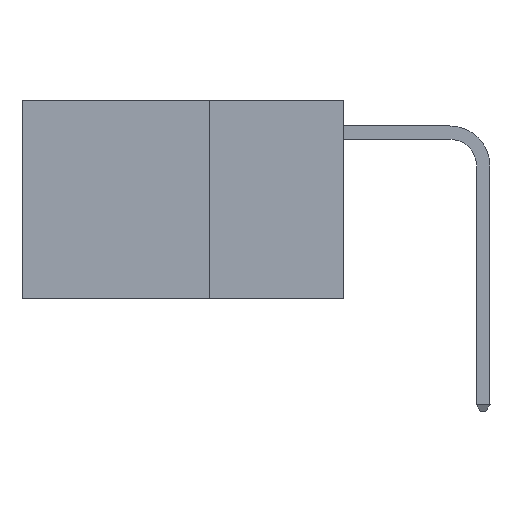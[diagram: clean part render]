
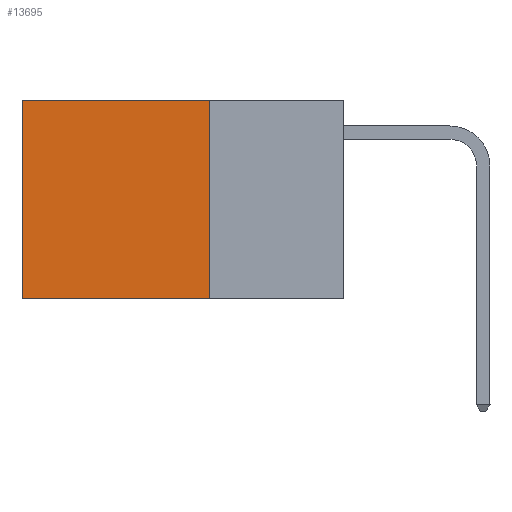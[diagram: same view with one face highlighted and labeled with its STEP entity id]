
A CAD part, left-side view. The second image highlights one B-rep face of the part: STEP entity #13695.
In plain terms, the highlighted planar face has unit normal (-1, 0, 0).
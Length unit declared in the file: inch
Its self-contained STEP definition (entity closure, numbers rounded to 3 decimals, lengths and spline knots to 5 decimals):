
#112 = VERTEX_POINT ( 'NONE', #3326 ) ;
#118 = VECTOR ( 'NONE', #8805, 39.37008 ) ;
#427 = VERTEX_POINT ( 'NONE', #9877 ) ;
#803 = LINE ( 'NONE', #5636, #10724 ) ;
#1195 = ORIENTED_EDGE ( 'NONE', *, *, #6217, .F. ) ;
#2635 = ORIENTED_EDGE ( 'NONE', *, *, #12765, .T. ) ;
#3182 = VERTEX_POINT ( 'NONE', #5630 ) ;
#3326 = CARTESIAN_POINT ( 'NONE',  ( 0.2625, 0.6, 0. ) ) ;
#4010 = DIRECTION ( 'NONE',  ( 1., 0., 0. ) ) ;
#4047 = VERTEX_POINT ( 'NONE', #9725 ) ;
#4146 = CARTESIAN_POINT ( 'NONE',  ( 0.2625, 0.25, 0. ) ) ;
#4190 = LINE ( 'NONE', #5335, #9816 ) ;
#4846 = EDGE_CURVE ( 'NONE', #112, #4047, #803, .T. ) ;
#5148 = PLANE ( 'NONE',  #12295 ) ;
#5335 = CARTESIAN_POINT ( 'NONE',  ( 0.2625, 0.25, 0. ) ) ;
#5630 = CARTESIAN_POINT ( 'NONE',  ( 0.2625, 0.25, 0. ) ) ;
#5636 = CARTESIAN_POINT ( 'NONE',  ( 0.2625, 0.6, 0. ) ) ;
#6105 = ORIENTED_EDGE ( 'NONE', *, *, #8054, .F. ) ;
#6217 = EDGE_CURVE ( 'NONE', #3182, #427, #14598, .T. ) ;
#6706 = LINE ( 'NONE', #13951, #11980 ) ;
#8054 = EDGE_CURVE ( 'NONE', #427, #4047, #6706, .T. ) ;
#8805 = DIRECTION ( 'NONE',  ( 0., 0., -1. ) ) ;
#8926 = DIRECTION ( 'NONE',  ( 0., 1., 0. ) ) ;
#9725 = CARTESIAN_POINT ( 'NONE',  ( 0.2625, 0.6, -0.37 ) ) ;
#9816 = VECTOR ( 'NONE', #8926, 39.37008 ) ;
#9877 = CARTESIAN_POINT ( 'NONE',  ( 0.2625, 0.25, -0.37 ) ) ;
#10352 = DIRECTION ( 'NONE',  ( 0., 0., -1. ) ) ;
#10724 = VECTOR ( 'NONE', #10352, 39.37008 ) ;
#11732 = EDGE_LOOP ( 'NONE', ( #14172, #6105, #1195, #2635 ) ) ;
#11980 = VECTOR ( 'NONE', #15178, 39.37008 ) ;
#12159 = FACE_OUTER_BOUND ( 'NONE', #11732, .T. ) ;
#12237 = DIRECTION ( 'NONE',  ( 0., 0., -1. ) ) ;
#12295 = AXIS2_PLACEMENT_3D ( 'NONE', #14542, #4010, #12237 ) ;
#12765 = EDGE_CURVE ( 'NONE', #3182, #112, #4190, .T. ) ;
#13695 = ADVANCED_FACE ( 'NONE', ( #12159 ), #5148, .F. ) ;
#13951 = CARTESIAN_POINT ( 'NONE',  ( 0.2625, 0.25, -0.37 ) ) ;
#14172 = ORIENTED_EDGE ( 'NONE', *, *, #4846, .T. ) ;
#14542 = CARTESIAN_POINT ( 'NONE',  ( 0.2625, 0.25, 0. ) ) ;
#14598 = LINE ( 'NONE', #4146, #118 ) ;
#15178 = DIRECTION ( 'NONE',  ( 0., 1., 0. ) ) ;
